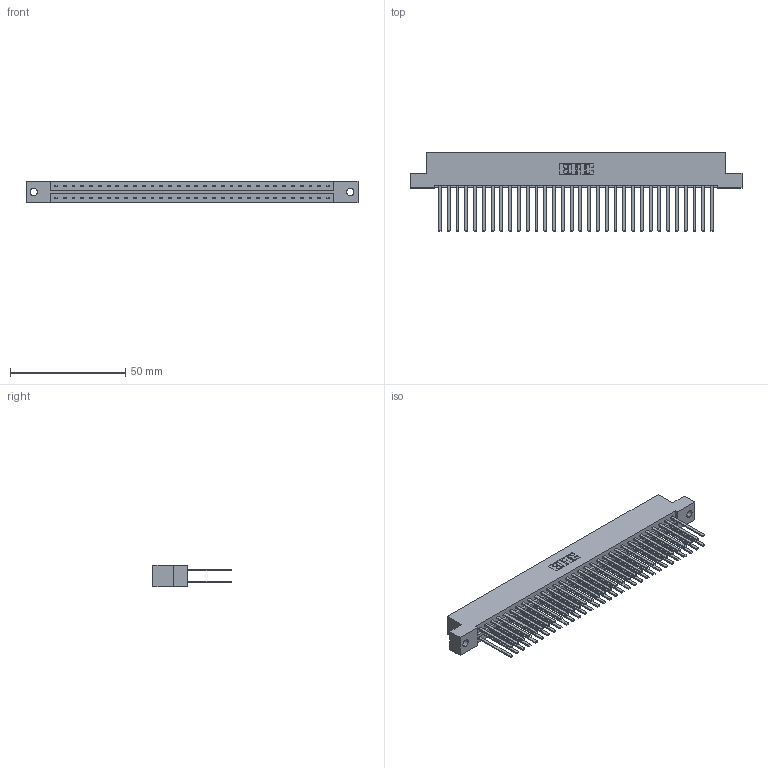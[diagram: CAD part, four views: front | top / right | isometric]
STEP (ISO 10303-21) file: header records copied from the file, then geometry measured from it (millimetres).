
FILE_DESCRIPTION (( 'STEP AP203' ), '1' );
FILE_NAME ('379-064-544-202.STEP', '2020-02-26T18:55:34', ( '' ), ( '' ), 'SwSTEP 2.0', 'SolidWorks 2016', '' );
FILE_SCHEMA (( 'CONFIG_CONTROL_DESIGN' ));
Length unit declared in the file: inch
Products named in the file (3): 379 Part_Flush - .128 Dia; 379-064-544-202; 345-292-001_345-293-144
Assembly tree (65 placements, depth 2):
  379-064-544-202
    379 Part_Flush - .128 Dia
    345-292-001_345-293-144  x64
Bounding box: 144.15 x 33.96 x 9.53 mm (x, y, z)
Volume: 16095.1 mm3; surface area: 20650.8 mm2
Topology: 65 solids, 65 shells, 3058 faces, 9079 edges, 5966 vertices
Faces by surface type: plane 2118, cylinder 940
Entity records: 21699 total; most frequent: CARTESIAN_POINT 3606, ORIENTED_EDGE 3542, DIRECTION 3095, EDGE_CURVE 1771, VECTOR 1647, LINE 1647, VERTEX_POINT 1178, AXIS2_PLACEMENT_3D 724
